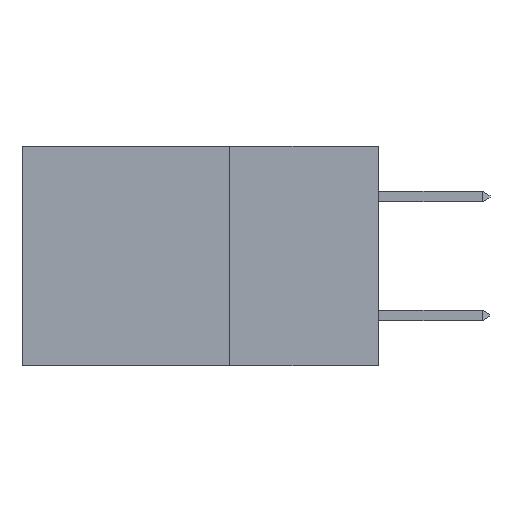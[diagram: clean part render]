
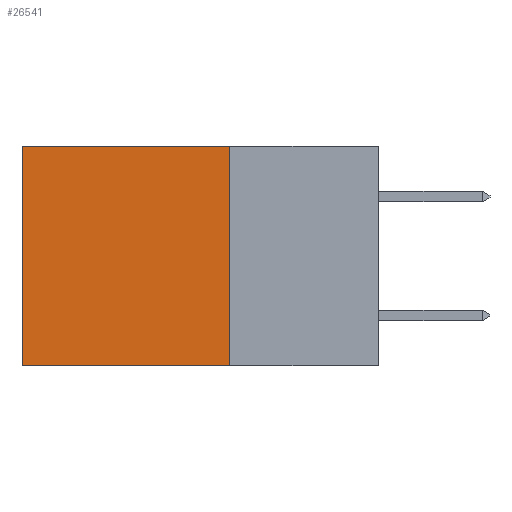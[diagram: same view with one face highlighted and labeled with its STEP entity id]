
A CAD part, left-side view. The second image highlights one B-rep face of the part: STEP entity #26541.
In plain terms, the highlighted planar face has unit normal (-1, 0, 0).
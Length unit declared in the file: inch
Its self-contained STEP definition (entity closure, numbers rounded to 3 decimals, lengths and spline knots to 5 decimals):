
#2946 = VECTOR ( 'NONE', #8502, 39.37008 ) ;
#3188 = CARTESIAN_POINT ( 'NONE',  ( 0.298, 0.25, 0. ) ) ;
#3277 = VERTEX_POINT ( 'NONE', #10015 ) ;
#3812 = EDGE_CURVE ( 'NONE', #3277, #23690, #8641, .T. ) ;
#4455 = DIRECTION ( 'NONE',  ( 0., 0., -1. ) ) ;
#4557 = ORIENTED_EDGE ( 'NONE', *, *, #27021, .T. ) ;
#6064 = CARTESIAN_POINT ( 'NONE',  ( 0.298, 0.25, 0. ) ) ;
#6880 = VECTOR ( 'NONE', #4455, 39.37008 ) ;
#7073 = EDGE_LOOP ( 'NONE', ( #17263, #12788, #14084, #4557 ) ) ;
#7723 = CARTESIAN_POINT ( 'NONE',  ( 0.298, 0.25, 0. ) ) ;
#8030 = VERTEX_POINT ( 'NONE', #15992 ) ;
#8502 = DIRECTION ( 'NONE',  ( 0., 1., 0. ) ) ;
#8641 = LINE ( 'NONE', #16371, #2946 ) ;
#10015 = CARTESIAN_POINT ( 'NONE',  ( 0.298, 0.25, -0.37 ) ) ;
#10081 = EDGE_CURVE ( 'NONE', #8030, #23690, #12159, .T. ) ;
#10483 = DIRECTION ( 'NONE',  ( 1., 0., 0. ) ) ;
#10560 = LINE ( 'NONE', #17240, #6880 ) ;
#12159 = LINE ( 'NONE', #18238, #17844 ) ;
#12788 = ORIENTED_EDGE ( 'NONE', *, *, #3812, .F. ) ;
#12878 = VECTOR ( 'NONE', #14022, 39.37008 ) ;
#13110 = CARTESIAN_POINT ( 'NONE',  ( 0.298, 0.6, -0.37 ) ) ;
#14022 = DIRECTION ( 'NONE',  ( 0., 1., 0. ) ) ;
#14084 = ORIENTED_EDGE ( 'NONE', *, *, #27281, .F. ) ;
#14089 = VERTEX_POINT ( 'NONE', #3188 ) ;
#14184 = LINE ( 'NONE', #7723, #12878 ) ;
#14934 = AXIS2_PLACEMENT_3D ( 'NONE', #6064, #10483, #25279 ) ;
#15992 = CARTESIAN_POINT ( 'NONE',  ( 0.298, 0.6, 0. ) ) ;
#16371 = CARTESIAN_POINT ( 'NONE',  ( 0.298, 0.25, -0.37 ) ) ;
#17240 = CARTESIAN_POINT ( 'NONE',  ( 0.298, 0.25, 0. ) ) ;
#17263 = ORIENTED_EDGE ( 'NONE', *, *, #10081, .T. ) ;
#17844 = VECTOR ( 'NONE', #26575, 39.37008 ) ;
#18238 = CARTESIAN_POINT ( 'NONE',  ( 0.298, 0.6, 0. ) ) ;
#23195 = PLANE ( 'NONE',  #14934 ) ;
#23690 = VERTEX_POINT ( 'NONE', #13110 ) ;
#25279 = DIRECTION ( 'NONE',  ( 0., 0., -1. ) ) ;
#25499 = FACE_OUTER_BOUND ( 'NONE', #7073, .T. ) ;
#26541 = ADVANCED_FACE ( 'NONE', ( #25499 ), #23195, .F. ) ;
#26575 = DIRECTION ( 'NONE',  ( 0., 0., -1. ) ) ;
#27021 = EDGE_CURVE ( 'NONE', #14089, #8030, #14184, .T. ) ;
#27281 = EDGE_CURVE ( 'NONE', #14089, #3277, #10560, .T. ) ;
